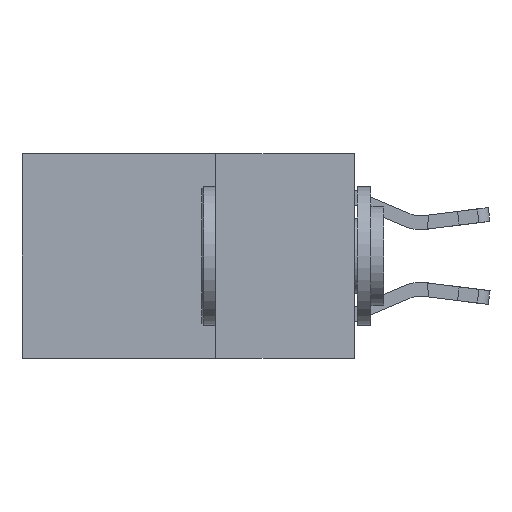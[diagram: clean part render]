
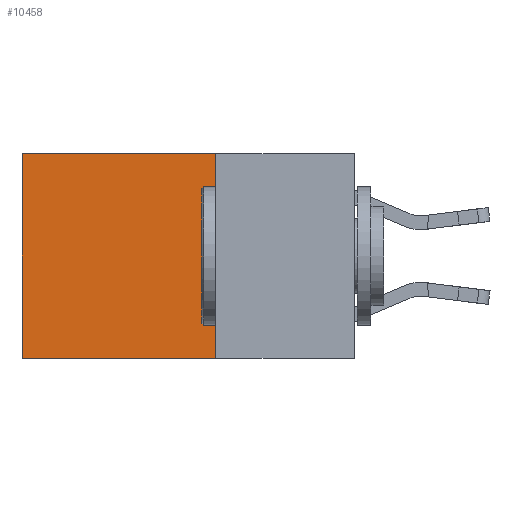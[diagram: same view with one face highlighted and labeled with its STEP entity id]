
A CAD part, left-side view. The second image highlights one B-rep face of the part: STEP entity #10458.
In plain terms, the highlighted planar face has unit normal (-1, 0, 0).
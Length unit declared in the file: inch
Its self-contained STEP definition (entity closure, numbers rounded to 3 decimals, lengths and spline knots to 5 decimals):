
#219 = VERTEX_POINT ( 'NONE', #8462 ) ;
#1383 = VERTEX_POINT ( 'NONE', #5560 ) ;
#1939 = LINE ( 'NONE', #9979, #2683 ) ;
#2114 = EDGE_LOOP ( 'NONE', ( #7320, #9000, #5533, #7871 ) ) ;
#2179 = VECTOR ( 'NONE', #2535, 39.37008 ) ;
#2400 = VECTOR ( 'NONE', #10198, 39.37008 ) ;
#2458 = EDGE_CURVE ( 'NONE', #4673, #1383, #2515, .T. ) ;
#2515 = LINE ( 'NONE', #6779, #9668 ) ;
#2535 = DIRECTION ( 'NONE',  ( 0., 0., -1. ) ) ;
#2683 = VECTOR ( 'NONE', #11785, 39.37008 ) ;
#3019 = CARTESIAN_POINT ( 'NONE',  ( 0.2625, 0.6, 0. ) ) ;
#3045 = CARTESIAN_POINT ( 'NONE',  ( 0.2625, 0.25, 0. ) ) ;
#4673 = VERTEX_POINT ( 'NONE', #3045 ) ;
#5533 = ORIENTED_EDGE ( 'NONE', *, *, #2458, .F. ) ;
#5560 = CARTESIAN_POINT ( 'NONE',  ( 0.2625, 0.25, -0.37 ) ) ;
#5963 = FACE_OUTER_BOUND ( 'NONE', #2114, .T. ) ;
#6560 = EDGE_CURVE ( 'NONE', #8223, #219, #11465, .T. ) ;
#6779 = CARTESIAN_POINT ( 'NONE',  ( 0.2625, 0.25, 0. ) ) ;
#7014 = AXIS2_PLACEMENT_3D ( 'NONE', #7649, #9758, #8719 ) ;
#7320 = ORIENTED_EDGE ( 'NONE', *, *, #6560, .T. ) ;
#7486 = LINE ( 'NONE', #12284, #2400 ) ;
#7649 = CARTESIAN_POINT ( 'NONE',  ( 0.2625, 0.25, 0. ) ) ;
#7776 = DIRECTION ( 'NONE',  ( 0., 0., -1. ) ) ;
#7871 = ORIENTED_EDGE ( 'NONE', *, *, #10594, .T. ) ;
#8223 = VERTEX_POINT ( 'NONE', #9307 ) ;
#8462 = CARTESIAN_POINT ( 'NONE',  ( 0.2625, 0.6, -0.37 ) ) ;
#8719 = DIRECTION ( 'NONE',  ( 0., 0., -1. ) ) ;
#9000 = ORIENTED_EDGE ( 'NONE', *, *, #10320, .F. ) ;
#9307 = CARTESIAN_POINT ( 'NONE',  ( 0.2625, 0.6, 0. ) ) ;
#9668 = VECTOR ( 'NONE', #7776, 39.37008 ) ;
#9758 = DIRECTION ( 'NONE',  ( 1., 0., 0. ) ) ;
#9979 = CARTESIAN_POINT ( 'NONE',  ( 0.2625, 0.25, 0. ) ) ;
#10198 = DIRECTION ( 'NONE',  ( 0., 1., 0. ) ) ;
#10320 = EDGE_CURVE ( 'NONE', #1383, #219, #7486, .T. ) ;
#10458 = ADVANCED_FACE ( 'NONE', ( #5963 ), #12718, .F. ) ;
#10594 = EDGE_CURVE ( 'NONE', #4673, #8223, #1939, .T. ) ;
#11465 = LINE ( 'NONE', #3019, #2179 ) ;
#11785 = DIRECTION ( 'NONE',  ( 0., 1., 0. ) ) ;
#12284 = CARTESIAN_POINT ( 'NONE',  ( 0.2625, 0.25, -0.37 ) ) ;
#12718 = PLANE ( 'NONE',  #7014 ) ;
